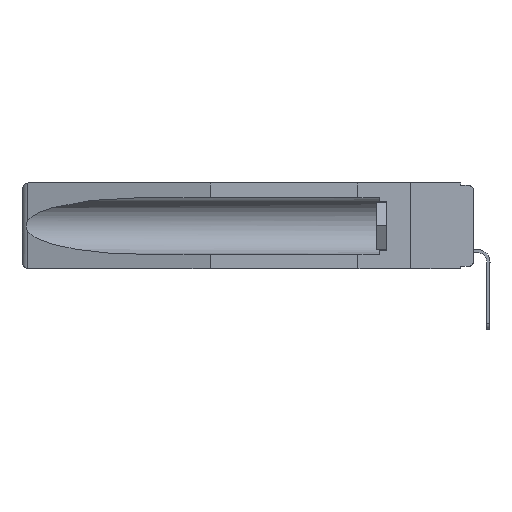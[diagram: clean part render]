
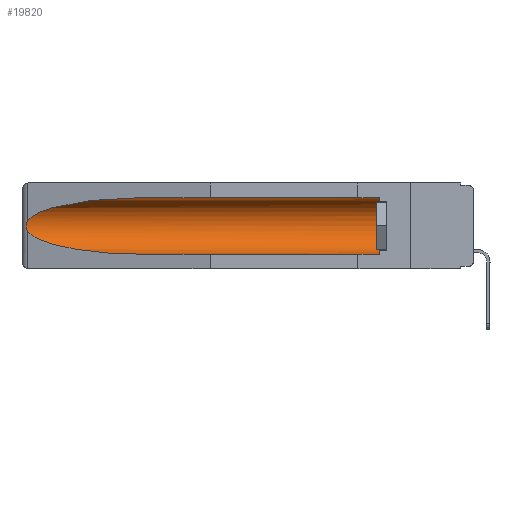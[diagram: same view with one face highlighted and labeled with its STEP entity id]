
A CAD part, left-side view. The second image highlights one B-rep face of the part: STEP entity #19820.
In plain terms, the highlighted cylindrical face has radius 2.857 mm (diameter 5.715 mm), a partial arc.
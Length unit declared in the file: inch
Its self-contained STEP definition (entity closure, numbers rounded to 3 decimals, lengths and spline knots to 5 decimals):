
#419 = ORIENTED_EDGE ( 'NONE', *, *, #11693, .T. ) ;
#1455 = VERTEX_POINT ( 'NONE', #5025 ) ;
#1731 = CARTESIAN_POINT ( 'NONE',  ( 0.155, -0.30754, -0.059 ) ) ;
#1937 = AXIS2_PLACEMENT_3D ( 'NONE', #4326, #14504, #4207 ) ;
#2279 = EDGE_CURVE ( 'NONE', #8055, #1455, #9864, .T. ) ;
#2379 = CARTESIAN_POINT ( 'NONE',  ( 0.2673, 1.5327, -0.16383 ) ) ;
#3487 = DIRECTION ( 'NONE',  ( 0., 0., 1. ) ) ;
#3822 = CARTESIAN_POINT ( 'NONE',  ( 0.155, 1.07973, -0.059 ) ) ;
#4207 = DIRECTION ( 'NONE',  ( 0., 0., 1. ) ) ;
#4326 = CARTESIAN_POINT ( 'NONE',  ( 0.155, -0.30754, -0.1715 ) ) ;
#4401 = CARTESIAN_POINT ( 'NONE',  ( 0.26597, 1.5296, -0.19026 ) ) ;
#4663 = CARTESIAN_POINT ( 'NONE',  ( 0.25451, 1.48313, -0.09465 ) ) ;
#4680 = CARTESIAN_POINT ( 'NONE',  ( 0.26537, 1.52718, -0.19328 ) ) ;
#5025 = CARTESIAN_POINT ( 'NONE',  ( 0.26537, 1.52718, -0.19328 ) ) ;
#5664 = EDGE_CURVE ( 'NONE', #10435, #8055, #10734, .T. ) ;
#6606 = CARTESIAN_POINT ( 'NONE',  ( 0.155, 0.126, -0.1715 ) ) ;
#6711 = CARTESIAN_POINT ( 'NONE',  ( 0.26597, 1.52961, -0.15275 ) ) ;
#6844 = CARTESIAN_POINT ( 'NONE',  ( 0.26655, 1.53094, -0.18657 ) ) ;
#6945 = CARTESIAN_POINT ( 'NONE',  ( 0.155, 1.07973, -0.284 ) ) ;
#7726 = LINE ( 'NONE', #1731, #19626 ) ;
#8055 = VERTEX_POINT ( 'NONE', #21120 ) ;
#8765 = LINE ( 'NONE', #12547, #24311 ) ;
#8887 = CARTESIAN_POINT ( 'NONE',  ( 0.2675, 1.53308, -0.17534 ) ) ;
#9864 = B_SPLINE_CURVE_WITH_KNOTS ( 'NONE', 3,
 ( #19049, #6711, #14979, #2379, #23265, #8887, #21211, #6844, #4401, #4680 ),
 .UNSPECIFIED., .F., .F.,
 ( 4, 2, 2, 2, 4 ),
 ( 0., 0.00029, 0.00058, 0.00087, 0.00117 ),
 .UNSPECIFIED. ) ;
#10015 = DIRECTION ( 'NONE',  ( 0., 1., 0. ) ) ;
#10435 = VERTEX_POINT ( 'NONE', #3822 ) ;
#10734 =( BOUNDED_CURVE ( )  B_SPLINE_CURVE ( 3, ( #11292, #16854, #4663, #17140 ),
 .UNSPECIFIED., .F., .T. ) 
 B_SPLINE_CURVE_WITH_KNOTS ( ( 4, 4 ),
 ( 4.71239, 6.08839 ),
 .UNSPECIFIED. ) 
 CURVE ( )  GEOMETRIC_REPRESENTATION_ITEM ( )  RATIONAL_B_SPLINE_CURVE ( ( 1., 0.848, 0.848, 1. ) ) 
 REPRESENTATION_ITEM ( '' )  );
#11292 = CARTESIAN_POINT ( 'NONE',  ( 0.155, 1.07973, -0.059 ) ) ;
#11693 = EDGE_CURVE ( 'NONE', #23749, #10435, #7726, .T. ) ;
#12319 = CIRCLE ( 'NONE', #24480, 0.1125 ) ;
#12547 = CARTESIAN_POINT ( 'NONE',  ( 0.155, -0.30754, -0.284 ) ) ;
#12826 = DIRECTION ( 'NONE',  ( 0., 1., 0. ) ) ;
#12881 = EDGE_CURVE ( 'NONE', #1455, #19662, #14535, .T. ) ;
#13709 = ORIENTED_EDGE ( 'NONE', *, *, #15989, .F. ) ;
#14504 = DIRECTION ( 'NONE',  ( 0., 1., 0. ) ) ;
#14535 =( BOUNDED_CURVE ( )  B_SPLINE_CURVE ( 3, ( #19669, #21973, #17500, #25924 ),
 .UNSPECIFIED., .F., .T. ) 
 B_SPLINE_CURVE_WITH_KNOTS ( ( 4, 4 ),
 ( 0.1948, 1.5708 ),
 .UNSPECIFIED. ) 
 CURVE ( )  GEOMETRIC_REPRESENTATION_ITEM ( )  RATIONAL_B_SPLINE_CURVE ( ( 1., 0.848, 0.848, 1. ) ) 
 REPRESENTATION_ITEM ( '' )  );
#14545 = EDGE_CURVE ( 'NONE', #14669, #23749, #12319, .T. ) ;
#14669 = VERTEX_POINT ( 'NONE', #16232 ) ;
#14979 = CARTESIAN_POINT ( 'NONE',  ( 0.26654, 1.53092, -0.15636 ) ) ;
#15989 = EDGE_CURVE ( 'NONE', #14669, #19662, #8765, .T. ) ;
#16232 = CARTESIAN_POINT ( 'NONE',  ( 0.155, 0.126, -0.284 ) ) ;
#16593 = CARTESIAN_POINT ( 'NONE',  ( 0.155, 0.126, -0.059 ) ) ;
#16854 = CARTESIAN_POINT ( 'NONE',  ( 0.21114, 1.30732, -0.059 ) ) ;
#17140 = CARTESIAN_POINT ( 'NONE',  ( 0.26537, 1.52718, -0.14972 ) ) ;
#17500 = CARTESIAN_POINT ( 'NONE',  ( 0.21114, 1.30732, -0.284 ) ) ;
#18210 = ORIENTED_EDGE ( 'NONE', *, *, #5664, .T. ) ;
#19049 = CARTESIAN_POINT ( 'NONE',  ( 0.26537, 1.52718, -0.14972 ) ) ;
#19307 = EDGE_LOOP ( 'NONE', ( #18210, #22775, #26277, #13709, #21697, #419 ) ) ;
#19626 = VECTOR ( 'NONE', #10015, 39.37008 ) ;
#19662 = VERTEX_POINT ( 'NONE', #6945 ) ;
#19669 = CARTESIAN_POINT ( 'NONE',  ( 0.26537, 1.52718, -0.19328 ) ) ;
#19820 = ADVANCED_FACE ( 'NONE', ( #21136 ), #25499, .F. ) ;
#21120 = CARTESIAN_POINT ( 'NONE',  ( 0.26537, 1.52718, -0.14972 ) ) ;
#21136 = FACE_OUTER_BOUND ( 'NONE', #19307, .T. ) ;
#21211 = CARTESIAN_POINT ( 'NONE',  ( 0.2673, 1.53269, -0.17917 ) ) ;
#21697 = ORIENTED_EDGE ( 'NONE', *, *, #14545, .T. ) ;
#21973 = CARTESIAN_POINT ( 'NONE',  ( 0.25451, 1.48313, -0.24835 ) ) ;
#22068 = DIRECTION ( 'NONE',  ( 0., -1., 0. ) ) ;
#22775 = ORIENTED_EDGE ( 'NONE', *, *, #2279, .T. ) ;
#23265 = CARTESIAN_POINT ( 'NONE',  ( 0.2675, 1.53308, -0.16763 ) ) ;
#23749 = VERTEX_POINT ( 'NONE', #16593 ) ;
#24311 = VECTOR ( 'NONE', #12826, 39.37008 ) ;
#24480 = AXIS2_PLACEMENT_3D ( 'NONE', #6606, #22068, #3487 ) ;
#25499 = CYLINDRICAL_SURFACE ( 'NONE', #1937, 0.1125 ) ;
#25924 = CARTESIAN_POINT ( 'NONE',  ( 0.155, 1.07973, -0.284 ) ) ;
#26277 = ORIENTED_EDGE ( 'NONE', *, *, #12881, .T. ) ;
